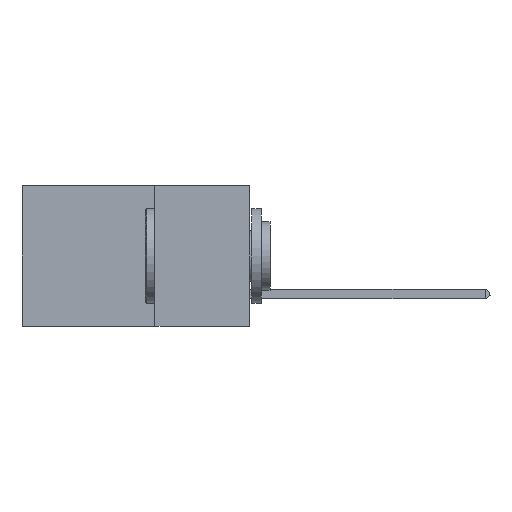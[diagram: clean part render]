
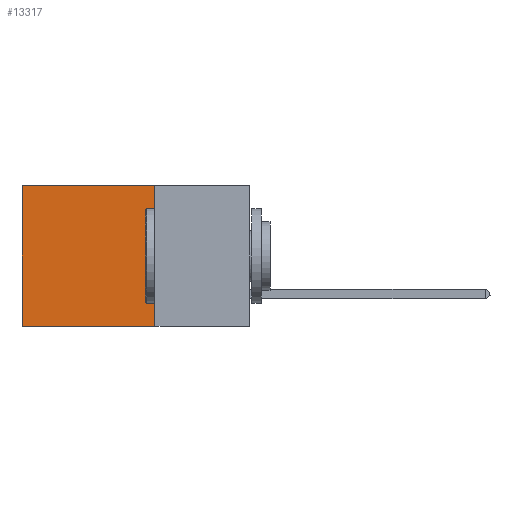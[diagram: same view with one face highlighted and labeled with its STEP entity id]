
A CAD part, left-side view. The second image highlights one B-rep face of the part: STEP entity #13317.
In plain terms, the highlighted planar face has unit normal (-1, 0, 0).
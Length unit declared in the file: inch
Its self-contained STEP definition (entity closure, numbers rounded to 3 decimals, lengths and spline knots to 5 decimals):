
#7 = EDGE_CURVE ( 'NONE', #4845, #25597, #3700, .T. ) ;
#1125 = EDGE_LOOP ( 'NONE', ( #1778, #17055, #16271, #2786 ) ) ;
#1778 = ORIENTED_EDGE ( 'NONE', *, *, #5777, .T. ) ;
#1783 = VECTOR ( 'NONE', #20600, 39.37008 ) ;
#2568 = CARTESIAN_POINT ( 'NONE',  ( 0.2875, 0.6, -0.37 ) ) ;
#2786 = ORIENTED_EDGE ( 'NONE', *, *, #4490, .T. ) ;
#3569 = DIRECTION ( 'NONE',  ( 0., 0., -1. ) ) ;
#3700 = LINE ( 'NONE', #18257, #19139 ) ;
#3926 = VERTEX_POINT ( 'NONE', #15491 ) ;
#4490 = EDGE_CURVE ( 'NONE', #4845, #3926, #5875, .T. ) ;
#4845 = VERTEX_POINT ( 'NONE', #20792 ) ;
#5344 = PLANE ( 'NONE',  #5491 ) ;
#5491 = AXIS2_PLACEMENT_3D ( 'NONE', #26550, #11954, #3569 ) ;
#5777 = EDGE_CURVE ( 'NONE', #3926, #6323, #10411, .T. ) ;
#5875 = LINE ( 'NONE', #27161, #6180 ) ;
#6107 = LINE ( 'NONE', #7941, #1783 ) ;
#6180 = VECTOR ( 'NONE', #10118, 39.37008 ) ;
#6323 = VERTEX_POINT ( 'NONE', #2568 ) ;
#7941 = CARTESIAN_POINT ( 'NONE',  ( 0.2875, 0.25, -0.37 ) ) ;
#8994 = DIRECTION ( 'NONE',  ( 0., 0., -1. ) ) ;
#10118 = DIRECTION ( 'NONE',  ( 0., 1., 0. ) ) ;
#10411 = LINE ( 'NONE', #13173, #27219 ) ;
#10445 = FACE_OUTER_BOUND ( 'NONE', #1125, .T. ) ;
#11954 = DIRECTION ( 'NONE',  ( 1., 0., 0. ) ) ;
#13173 = CARTESIAN_POINT ( 'NONE',  ( 0.2875, 0.6, 0. ) ) ;
#13317 = ADVANCED_FACE ( 'NONE', ( #10445 ), #5344, .F. ) ;
#15491 = CARTESIAN_POINT ( 'NONE',  ( 0.2875, 0.6, 0. ) ) ;
#16163 = DIRECTION ( 'NONE',  ( 0., 0., -1. ) ) ;
#16271 = ORIENTED_EDGE ( 'NONE', *, *, #7, .F. ) ;
#17055 = ORIENTED_EDGE ( 'NONE', *, *, #22449, .F. ) ;
#18257 = CARTESIAN_POINT ( 'NONE',  ( 0.2875, 0.25, 0. ) ) ;
#19139 = VECTOR ( 'NONE', #16163, 39.37008 ) ;
#20600 = DIRECTION ( 'NONE',  ( 0., 1., 0. ) ) ;
#20792 = CARTESIAN_POINT ( 'NONE',  ( 0.2875, 0.25, 0. ) ) ;
#22449 = EDGE_CURVE ( 'NONE', #25597, #6323, #6107, .T. ) ;
#25597 = VERTEX_POINT ( 'NONE', #25920 ) ;
#25920 = CARTESIAN_POINT ( 'NONE',  ( 0.2875, 0.25, -0.37 ) ) ;
#26550 = CARTESIAN_POINT ( 'NONE',  ( 0.2875, 0.25, 0. ) ) ;
#27161 = CARTESIAN_POINT ( 'NONE',  ( 0.2875, 0.25, 0. ) ) ;
#27219 = VECTOR ( 'NONE', #8994, 39.37008 ) ;
